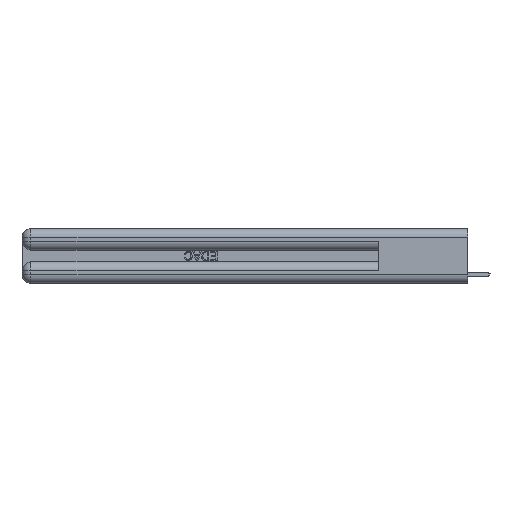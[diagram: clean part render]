
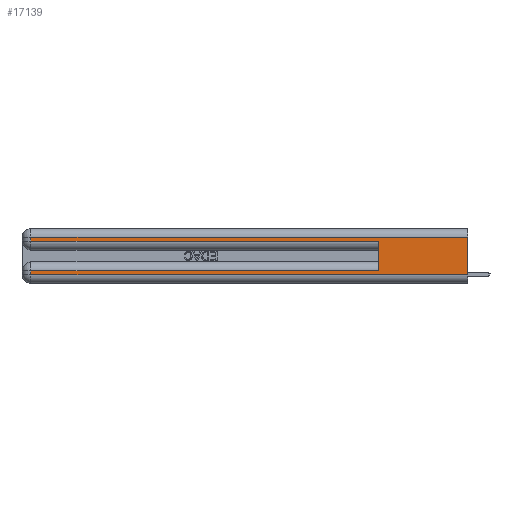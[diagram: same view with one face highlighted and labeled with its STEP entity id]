
A CAD part, left-side view. The second image highlights one B-rep face of the part: STEP entity #17139.
In plain terms, the highlighted planar face has unit normal (-1, 0, 0).
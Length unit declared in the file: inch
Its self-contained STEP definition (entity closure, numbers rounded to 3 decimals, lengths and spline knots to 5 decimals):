
#477 = CARTESIAN_POINT ( 'NONE',  ( 0., 0., 0.06 ) ) ;
#478 = CARTESIAN_POINT ( 'NONE',  ( 0., 0., 0.37 ) ) ;
#819 = CARTESIAN_POINT ( 'NONE',  ( 0., 0., 0.37 ) ) ;
#997 = VECTOR ( 'NONE', #26912, 39.37008 ) ;
#1310 = FACE_OUTER_BOUND ( 'NONE', #27061, .T. ) ;
#2078 = ORIENTED_EDGE ( 'NONE', *, *, #28095, .T. ) ;
#2694 = DIRECTION ( 'NONE',  ( 0., -1., 0. ) ) ;
#3224 = DIRECTION ( 'NONE',  ( 0., 0., -1. ) ) ;
#3664 = ORIENTED_EDGE ( 'NONE', *, *, #20126, .T. ) ;
#3689 = VECTOR ( 'NONE', #21010, 39.37008 ) ;
#3751 = VERTEX_POINT ( 'NONE', #22140 ) ;
#3934 = CARTESIAN_POINT ( 'NONE',  ( 0., 2.94, 0.06 ) ) ;
#4034 = LINE ( 'NONE', #477, #12296 ) ;
#4087 = EDGE_CURVE ( 'NONE', #3751, #9544, #18711, .T. ) ;
#4125 = CARTESIAN_POINT ( 'NONE',  ( 0., 0., 0.085 ) ) ;
#5594 = EDGE_CURVE ( 'NONE', #9544, #19824, #12627, .T. ) ;
#6396 = VECTOR ( 'NONE', #12247, 39.37008 ) ;
#7064 = PLANE ( 'NONE',  #7641 ) ;
#7334 = CARTESIAN_POINT ( 'NONE',  ( 0., 2.94, 0.37 ) ) ;
#7410 = VECTOR ( 'NONE', #11890, 39.37008 ) ;
#7491 = VERTEX_POINT ( 'NONE', #8698 ) ;
#7641 = AXIS2_PLACEMENT_3D ( 'NONE', #819, #9757, #23150 ) ;
#7895 = CARTESIAN_POINT ( 'NONE',  ( 0., 0.6, 0.145 ) ) ;
#8329 = VERTEX_POINT ( 'NONE', #24382 ) ;
#8546 = ORIENTED_EDGE ( 'NONE', *, *, #23259, .F. ) ;
#8698 = CARTESIAN_POINT ( 'NONE',  ( 0., 0., 0.31 ) ) ;
#9544 = VERTEX_POINT ( 'NONE', #23882 ) ;
#9757 = DIRECTION ( 'NONE',  ( 1., 0., 0. ) ) ;
#9824 = LINE ( 'NONE', #27293, #7410 ) ;
#9991 = CARTESIAN_POINT ( 'NONE',  ( 0., 0., 0.285 ) ) ;
#10607 = ORIENTED_EDGE ( 'NONE', *, *, #5594, .T. ) ;
#10830 = ORIENTED_EDGE ( 'NONE', *, *, #21621, .T. ) ;
#11486 = CARTESIAN_POINT ( 'NONE',  ( 0., 2.94, 0.37 ) ) ;
#11546 = ORIENTED_EDGE ( 'NONE', *, *, #11874, .F. ) ;
#11562 = EDGE_CURVE ( 'NONE', #26297, #18913, #22938, .T. ) ;
#11820 = VERTEX_POINT ( 'NONE', #22715 ) ;
#11874 = EDGE_CURVE ( 'NONE', #7491, #11820, #12292, .T. ) ;
#11890 = DIRECTION ( 'NONE',  ( 0., 1., 0. ) ) ;
#12245 = LINE ( 'NONE', #4125, #6396 ) ;
#12247 = DIRECTION ( 'NONE',  ( 0., 1., 0. ) ) ;
#12292 = LINE ( 'NONE', #478, #997 ) ;
#12296 = VECTOR ( 'NONE', #2694, 39.37008 ) ;
#12401 = DIRECTION ( 'NONE',  ( 0., 0., 1. ) ) ;
#12627 = LINE ( 'NONE', #9991, #3689 ) ;
#13030 = VECTOR ( 'NONE', #12401, 39.37008 ) ;
#13428 = CARTESIAN_POINT ( 'NONE',  ( 0., 0.6, 0.285 ) ) ;
#17040 = ORIENTED_EDGE ( 'NONE', *, *, #4087, .T. ) ;
#17139 = ADVANCED_FACE ( 'NONE', ( #1310 ), #7064, .F. ) ;
#18711 = LINE ( 'NONE', #11486, #24862 ) ;
#18913 = VERTEX_POINT ( 'NONE', #3934 ) ;
#19824 = VERTEX_POINT ( 'NONE', #13428 ) ;
#20126 = EDGE_CURVE ( 'NONE', #8329, #26297, #12245, .T. ) ;
#21010 = DIRECTION ( 'NONE',  ( 0., -1., 0. ) ) ;
#21621 = EDGE_CURVE ( 'NONE', #18913, #11820, #4034, .T. ) ;
#22140 = CARTESIAN_POINT ( 'NONE',  ( 0., 2.94, 0.31 ) ) ;
#22665 = DIRECTION ( 'NONE',  ( 0., 0., -1. ) ) ;
#22715 = CARTESIAN_POINT ( 'NONE',  ( 0., 0., 0.06 ) ) ;
#22938 = LINE ( 'NONE', #7334, #28048 ) ;
#23042 = CARTESIAN_POINT ( 'NONE',  ( 0., 2.94, 0.085 ) ) ;
#23150 = DIRECTION ( 'NONE',  ( 0., 0., -1. ) ) ;
#23259 = EDGE_CURVE ( 'NONE', #8329, #19824, #24008, .T. ) ;
#23467 = ORIENTED_EDGE ( 'NONE', *, *, #11562, .T. ) ;
#23882 = CARTESIAN_POINT ( 'NONE',  ( 0., 2.94, 0.285 ) ) ;
#24008 = LINE ( 'NONE', #7895, #13030 ) ;
#24382 = CARTESIAN_POINT ( 'NONE',  ( 0., 0.6, 0.085 ) ) ;
#24862 = VECTOR ( 'NONE', #3224, 39.37008 ) ;
#26297 = VERTEX_POINT ( 'NONE', #23042 ) ;
#26912 = DIRECTION ( 'NONE',  ( 0., 0., -1. ) ) ;
#27061 = EDGE_LOOP ( 'NONE', ( #11546, #2078, #17040, #10607, #8546, #3664, #23467, #10830 ) ) ;
#27293 = CARTESIAN_POINT ( 'NONE',  ( 0., 0., 0.31 ) ) ;
#28048 = VECTOR ( 'NONE', #22665, 39.37008 ) ;
#28095 = EDGE_CURVE ( 'NONE', #7491, #3751, #9824, .T. ) ;
